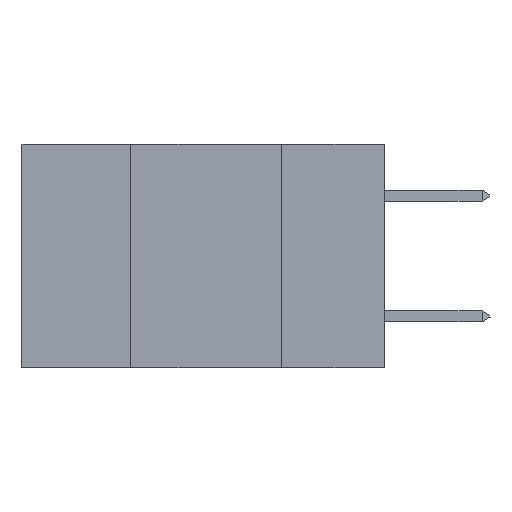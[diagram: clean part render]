
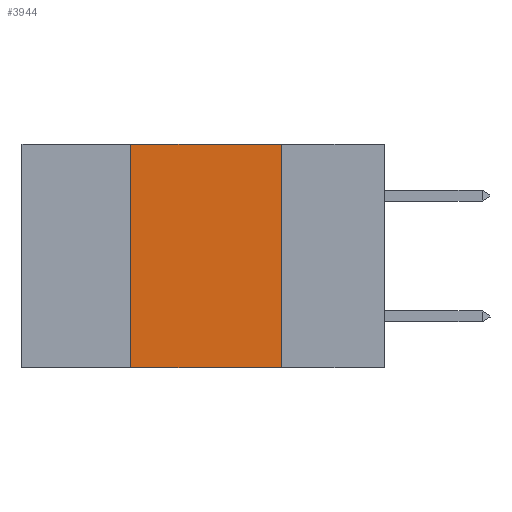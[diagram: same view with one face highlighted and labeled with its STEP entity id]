
A CAD part, left-side view. The second image highlights one B-rep face of the part: STEP entity #3944.
In plain terms, the highlighted planar face has unit normal (-1, 0, 0).
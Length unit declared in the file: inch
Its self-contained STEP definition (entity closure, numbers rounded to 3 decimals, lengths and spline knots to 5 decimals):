
#194 = CARTESIAN_POINT ( 'NONE',  ( 0., 0.6, 0. ) ) ;
#253 = VECTOR ( 'NONE', #15165, 39.37008 ) ;
#536 = EDGE_CURVE ( 'NONE', #18464, #18329, #3824, .T. ) ;
#623 = CARTESIAN_POINT ( 'NONE',  ( 0., 0.6, 0. ) ) ;
#733 = LINE ( 'NONE', #5343, #14323 ) ;
#839 = VECTOR ( 'NONE', #2112, 39.37008 ) ;
#2112 = DIRECTION ( 'NONE',  ( 0., -1., 0. ) ) ;
#3347 = CARTESIAN_POINT ( 'NONE',  ( 0., 0.42, -0.37 ) ) ;
#3824 = LINE ( 'NONE', #13158, #12415 ) ;
#3944 = ADVANCED_FACE ( 'NONE', ( #17736 ), #16483, .F. ) ;
#4471 = CARTESIAN_POINT ( 'NONE',  ( 0., 0.6, -0.37 ) ) ;
#5009 = EDGE_CURVE ( 'NONE', #18464, #10056, #11363, .T. ) ;
#5343 = CARTESIAN_POINT ( 'NONE',  ( 0., 0.17, 0. ) ) ;
#5803 = DIRECTION ( 'NONE',  ( 0., 0., 1. ) ) ;
#5837 = DIRECTION ( 'NONE',  ( 0., 0., -1. ) ) ;
#6328 = CARTESIAN_POINT ( 'NONE',  ( 0., 0.42, 0. ) ) ;
#7145 = DIRECTION ( 'NONE',  ( 0., 0., -1. ) ) ;
#7512 = LINE ( 'NONE', #194, #839 ) ;
#7590 = ORIENTED_EDGE ( 'NONE', *, *, #536, .F. ) ;
#7986 = EDGE_CURVE ( 'NONE', #18329, #8465, #7512, .T. ) ;
#8277 = CARTESIAN_POINT ( 'NONE',  ( 0., 0.17, -0.37 ) ) ;
#8465 = VERTEX_POINT ( 'NONE', #20547 ) ;
#9987 = ORIENTED_EDGE ( 'NONE', *, *, #13125, .F. ) ;
#10056 = VERTEX_POINT ( 'NONE', #8277 ) ;
#11363 = LINE ( 'NONE', #4471, #253 ) ;
#12415 = VECTOR ( 'NONE', #5803, 39.37008 ) ;
#13125 = EDGE_CURVE ( 'NONE', #8465, #10056, #733, .T. ) ;
#13158 = CARTESIAN_POINT ( 'NONE',  ( 0., 0.42, 0. ) ) ;
#14323 = VECTOR ( 'NONE', #7145, 39.37008 ) ;
#14800 = DIRECTION ( 'NONE',  ( 1., 0., 0. ) ) ;
#15165 = DIRECTION ( 'NONE',  ( 0., -1., 0. ) ) ;
#15433 = AXIS2_PLACEMENT_3D ( 'NONE', #623, #14800, #5837 ) ;
#15949 = ORIENTED_EDGE ( 'NONE', *, *, #5009, .T. ) ;
#16483 = PLANE ( 'NONE',  #15433 ) ;
#17736 = FACE_OUTER_BOUND ( 'NONE', #21875, .T. ) ;
#18244 = ORIENTED_EDGE ( 'NONE', *, *, #7986, .F. ) ;
#18329 = VERTEX_POINT ( 'NONE', #6328 ) ;
#18464 = VERTEX_POINT ( 'NONE', #3347 ) ;
#20547 = CARTESIAN_POINT ( 'NONE',  ( 0., 0.17, 0. ) ) ;
#21875 = EDGE_LOOP ( 'NONE', ( #9987, #18244, #7590, #15949 ) ) ;
